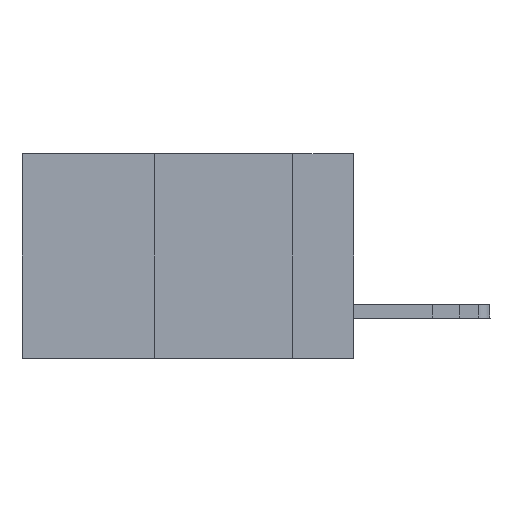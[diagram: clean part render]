
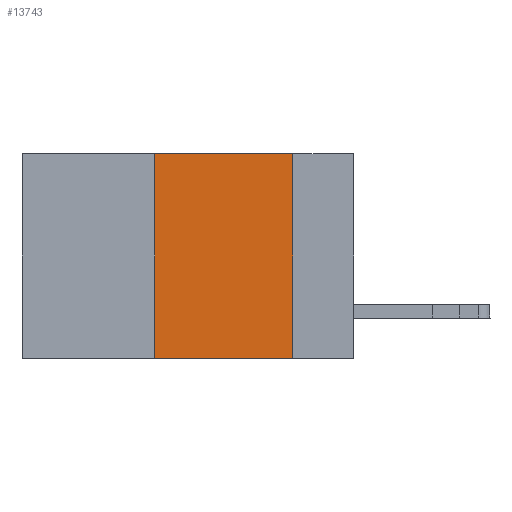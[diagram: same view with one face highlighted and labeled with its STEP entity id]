
A CAD part, left-side view. The second image highlights one B-rep face of the part: STEP entity #13743.
In plain terms, the highlighted planar face has unit normal (-1, 0, 0).
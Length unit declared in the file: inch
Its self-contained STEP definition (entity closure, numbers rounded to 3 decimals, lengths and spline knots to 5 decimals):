
#169 = VECTOR ( 'NONE', #26982, 39.37008 ) ;
#2085 = CARTESIAN_POINT ( 'NONE',  ( 0., 0.11, 0. ) ) ;
#3419 = EDGE_CURVE ( 'NONE', #5745, #25791, #14508, .T. ) ;
#4993 = CARTESIAN_POINT ( 'NONE',  ( 0., 0.36, 0. ) ) ;
#5282 = VERTEX_POINT ( 'NONE', #4993 ) ;
#5745 = VERTEX_POINT ( 'NONE', #28301 ) ;
#7887 = CARTESIAN_POINT ( 'NONE',  ( 0., 0.36, -0.37 ) ) ;
#8138 = VECTOR ( 'NONE', #14672, 39.37008 ) ;
#8515 = LINE ( 'NONE', #15016, #8138 ) ;
#8796 = EDGE_CURVE ( 'NONE', #5282, #5745, #29839, .T. ) ;
#9761 = PLANE ( 'NONE',  #32573 ) ;
#9998 = DIRECTION ( 'NONE',  ( 1., 0., 0. ) ) ;
#10562 = ORIENTED_EDGE ( 'NONE', *, *, #24574, .F. ) ;
#11050 = DIRECTION ( 'NONE',  ( 0., 0., 1. ) ) ;
#11321 = LINE ( 'NONE', #13595, #12166 ) ;
#12166 = VECTOR ( 'NONE', #11050, 39.37008 ) ;
#13595 = CARTESIAN_POINT ( 'NONE',  ( 0., 0.36, 0. ) ) ;
#13743 = ADVANCED_FACE ( 'NONE', ( #29323 ), #9761, .F. ) ;
#14508 = LINE ( 'NONE', #2085, #18621 ) ;
#14672 = DIRECTION ( 'NONE',  ( 0., -1., 0. ) ) ;
#15016 = CARTESIAN_POINT ( 'NONE',  ( 0., 0.6, -0.37 ) ) ;
#18621 = VECTOR ( 'NONE', #23171, 39.37008 ) ;
#20330 = ORIENTED_EDGE ( 'NONE', *, *, #8796, .F. ) ;
#20424 = CARTESIAN_POINT ( 'NONE',  ( 0., 0.11, -0.37 ) ) ;
#21924 = CARTESIAN_POINT ( 'NONE',  ( 0., 0.6, 0. ) ) ;
#22818 = VERTEX_POINT ( 'NONE', #7887 ) ;
#23171 = DIRECTION ( 'NONE',  ( 0., 0., -1. ) ) ;
#23985 = EDGE_CURVE ( 'NONE', #22818, #25791, #8515, .T. ) ;
#24574 = EDGE_CURVE ( 'NONE', #22818, #5282, #11321, .T. ) ;
#25647 = DIRECTION ( 'NONE',  ( 0., 0., -1. ) ) ;
#25785 = CARTESIAN_POINT ( 'NONE',  ( 0., 0.6, 0. ) ) ;
#25791 = VERTEX_POINT ( 'NONE', #20424 ) ;
#26491 = ORIENTED_EDGE ( 'NONE', *, *, #3419, .F. ) ;
#26982 = DIRECTION ( 'NONE',  ( 0., -1., 0. ) ) ;
#28301 = CARTESIAN_POINT ( 'NONE',  ( 0., 0.11, 0. ) ) ;
#29030 = ORIENTED_EDGE ( 'NONE', *, *, #23985, .T. ) ;
#29047 = EDGE_LOOP ( 'NONE', ( #26491, #20330, #10562, #29030 ) ) ;
#29323 = FACE_OUTER_BOUND ( 'NONE', #29047, .T. ) ;
#29839 = LINE ( 'NONE', #21924, #169 ) ;
#32573 = AXIS2_PLACEMENT_3D ( 'NONE', #25785, #9998, #25647 ) ;
